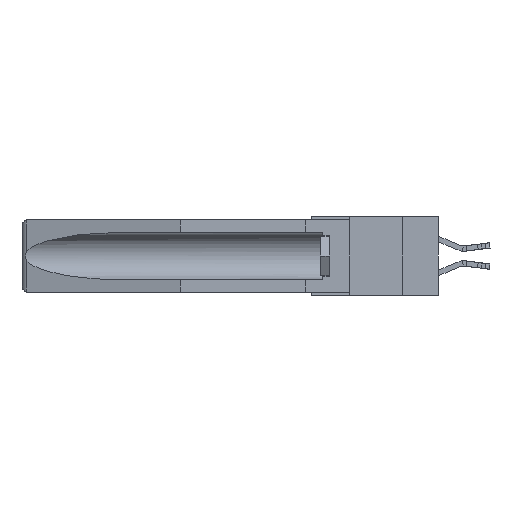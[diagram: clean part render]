
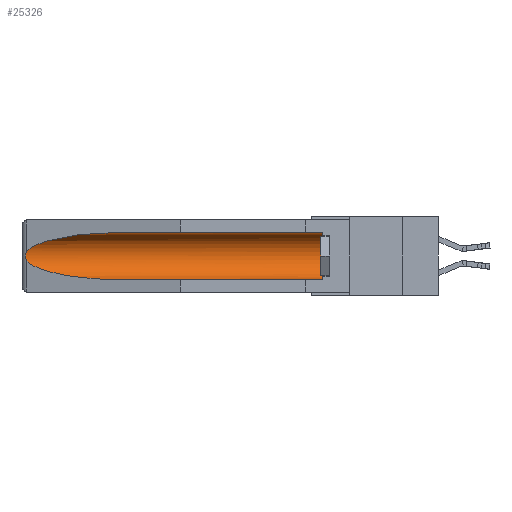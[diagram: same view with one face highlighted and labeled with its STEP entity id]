
A CAD part, left-side view. The second image highlights one B-rep face of the part: STEP entity #25326.
In plain terms, the highlighted cylindrical face has radius 2.857 mm (diameter 5.715 mm), a partial arc.
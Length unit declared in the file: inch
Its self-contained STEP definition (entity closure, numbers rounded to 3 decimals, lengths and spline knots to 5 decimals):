
#69 = CARTESIAN_POINT ( 'NONE',  ( 0.155, 1.07973, -0.059 ) ) ;
#409 = CARTESIAN_POINT ( 'NONE',  ( 0.2675, 1.53308, -0.17534 ) ) ;
#476 = CARTESIAN_POINT ( 'NONE',  ( 0.155, 1.07973, -0.059 ) ) ;
#667 = DIRECTION ( 'NONE',  ( 0., 1., 0. ) ) ;
#778 = CARTESIAN_POINT ( 'NONE',  ( 0.155, -0.30754, -0.1715 ) ) ;
#1036 = CARTESIAN_POINT ( 'NONE',  ( 0.155, 0.126, -0.1715 ) ) ;
#1735 = AXIS2_PLACEMENT_3D ( 'NONE', #1036, #20786, #10882 ) ;
#2035 = DIRECTION ( 'NONE',  ( 0., 1., 0. ) ) ;
#4528 = CARTESIAN_POINT ( 'NONE',  ( 0.21114, 1.30732, -0.284 ) ) ;
#4624 = EDGE_CURVE ( 'NONE', #7301, #29913, #8208, .T. ) ;
#4737 = ORIENTED_EDGE ( 'NONE', *, *, #4624, .T. ) ;
#5069 = EDGE_CURVE ( 'NONE', #26746, #24199, #16803, .T. ) ;
#6394 = VERTEX_POINT ( 'NONE', #24987 ) ;
#6667 = B_SPLINE_CURVE_WITH_KNOTS ( 'NONE', 3,
 ( #20358, #28198, #30405, #10354, #27793, #409, #17849, #18165, #20692, #13289 ),
 .UNSPECIFIED., .F., .F.,
 ( 4, 2, 2, 2, 4 ),
 ( 0., 0.00029, 0.00058, 0.00087, 0.00117 ),
 .UNSPECIFIED. ) ;
#6871 = CARTESIAN_POINT ( 'NONE',  ( 0.155, -0.30754, -0.059 ) ) ;
#7301 = VERTEX_POINT ( 'NONE', #31633 ) ;
#7436 = VECTOR ( 'NONE', #15417, 39.37008 ) ;
#8208 = LINE ( 'NONE', #6871, #11420 ) ;
#8222 = EDGE_CURVE ( 'NONE', #12777, #24199, #20693, .T. ) ;
#8373 = ORIENTED_EDGE ( 'NONE', *, *, #19238, .T. ) ;
#8782 = EDGE_LOOP ( 'NONE', ( #30784, #8373, #15806, #25128, #29616, #4737 ) ) ;
#9420 = CARTESIAN_POINT ( 'NONE',  ( 0.26537, 1.52718, -0.19328 ) ) ;
#10354 = CARTESIAN_POINT ( 'NONE',  ( 0.2673, 1.5327, -0.16383 ) ) ;
#10515 = CIRCLE ( 'NONE', #1735, 0.1125 ) ;
#10791 = CYLINDRICAL_SURFACE ( 'NONE', #28352, 0.1125 ) ;
#10882 = DIRECTION ( 'NONE',  ( 0., 0., 1. ) ) ;
#10991 = CARTESIAN_POINT ( 'NONE',  ( 0.155, 1.07973, -0.284 ) ) ;
#11420 = VECTOR ( 'NONE', #2035, 39.37008 ) ;
#12149 = CARTESIAN_POINT ( 'NONE',  ( 0.25451, 1.48313, -0.24835 ) ) ;
#12777 = VERTEX_POINT ( 'NONE', #32205 ) ;
#13289 = CARTESIAN_POINT ( 'NONE',  ( 0.26537, 1.52718, -0.19328 ) ) ;
#14996 = CARTESIAN_POINT ( 'NONE',  ( 0.25451, 1.48313, -0.09465 ) ) ;
#15417 = DIRECTION ( 'NONE',  ( 0., 1., 0. ) ) ;
#15806 = ORIENTED_EDGE ( 'NONE', *, *, #5069, .T. ) ;
#16803 =( BOUNDED_CURVE ( )  B_SPLINE_CURVE ( 3, ( #9420, #12149, #4528, #17135 ),
 .UNSPECIFIED., .F., .F. ) 
 B_SPLINE_CURVE_WITH_KNOTS ( ( 4, 4 ),
 ( 0.1948, 1.5708 ),
 .UNSPECIFIED. ) 
 CURVE ( )  GEOMETRIC_REPRESENTATION_ITEM ( )  RATIONAL_B_SPLINE_CURVE ( ( 1., 0.848, 0.848, 1. ) ) 
 REPRESENTATION_ITEM ( '' )  );
#17135 = CARTESIAN_POINT ( 'NONE',  ( 0.155, 1.07973, -0.284 ) ) ;
#17849 = CARTESIAN_POINT ( 'NONE',  ( 0.2673, 1.53269, -0.17917 ) ) ;
#17920 = CARTESIAN_POINT ( 'NONE',  ( 0.21114, 1.30732, -0.059 ) ) ;
#18165 = CARTESIAN_POINT ( 'NONE',  ( 0.26655, 1.53094, -0.18657 ) ) ;
#19238 = EDGE_CURVE ( 'NONE', #6394, #26746, #6667, .T. ) ;
#19799 = EDGE_CURVE ( 'NONE', #29913, #6394, #25962, .T. ) ;
#20300 = DIRECTION ( 'NONE',  ( 0., 0., 1. ) ) ;
#20358 = CARTESIAN_POINT ( 'NONE',  ( 0.26537, 1.52718, -0.14972 ) ) ;
#20692 = CARTESIAN_POINT ( 'NONE',  ( 0.26597, 1.5296, -0.19026 ) ) ;
#20693 = LINE ( 'NONE', #30358, #7436 ) ;
#20786 = DIRECTION ( 'NONE',  ( 0., -1., 0. ) ) ;
#21892 = EDGE_CURVE ( 'NONE', #12777, #7301, #10515, .T. ) ;
#22487 = CARTESIAN_POINT ( 'NONE',  ( 0.26537, 1.52718, -0.14972 ) ) ;
#24199 = VERTEX_POINT ( 'NONE', #10991 ) ;
#24987 = CARTESIAN_POINT ( 'NONE',  ( 0.26537, 1.52718, -0.14972 ) ) ;
#25128 = ORIENTED_EDGE ( 'NONE', *, *, #8222, .F. ) ;
#25326 = ADVANCED_FACE ( 'NONE', ( #29084 ), #10791, .F. ) ;
#25962 =( BOUNDED_CURVE ( )  B_SPLINE_CURVE ( 3, ( #476, #17920, #14996, #22487 ),
 .UNSPECIFIED., .F., .T. ) 
 B_SPLINE_CURVE_WITH_KNOTS ( ( 4, 4 ),
 ( 4.71239, 6.08839 ),
 .UNSPECIFIED. ) 
 CURVE ( )  GEOMETRIC_REPRESENTATION_ITEM ( )  RATIONAL_B_SPLINE_CURVE ( ( 1., 0.848, 0.848, 1. ) ) 
 REPRESENTATION_ITEM ( '' )  );
#26746 = VERTEX_POINT ( 'NONE', #27939 ) ;
#27793 = CARTESIAN_POINT ( 'NONE',  ( 0.2675, 1.53308, -0.16763 ) ) ;
#27939 = CARTESIAN_POINT ( 'NONE',  ( 0.26537, 1.52718, -0.19328 ) ) ;
#28198 = CARTESIAN_POINT ( 'NONE',  ( 0.26597, 1.52961, -0.15275 ) ) ;
#28352 = AXIS2_PLACEMENT_3D ( 'NONE', #778, #667, #20300 ) ;
#29084 = FACE_OUTER_BOUND ( 'NONE', #8782, .T. ) ;
#29616 = ORIENTED_EDGE ( 'NONE', *, *, #21892, .T. ) ;
#29913 = VERTEX_POINT ( 'NONE', #69 ) ;
#30358 = CARTESIAN_POINT ( 'NONE',  ( 0.155, -0.30754, -0.284 ) ) ;
#30405 = CARTESIAN_POINT ( 'NONE',  ( 0.26654, 1.53092, -0.15636 ) ) ;
#30784 = ORIENTED_EDGE ( 'NONE', *, *, #19799, .T. ) ;
#31633 = CARTESIAN_POINT ( 'NONE',  ( 0.155, 0.126, -0.059 ) ) ;
#32205 = CARTESIAN_POINT ( 'NONE',  ( 0.155, 0.126, -0.284 ) ) ;
